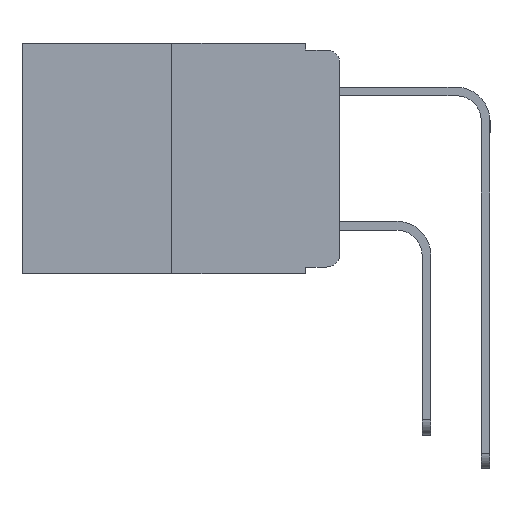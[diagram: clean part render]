
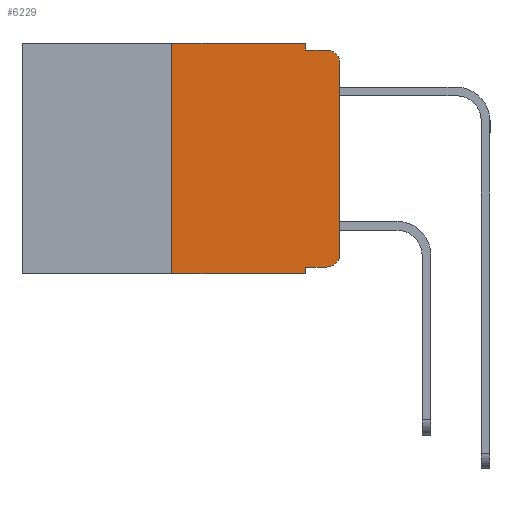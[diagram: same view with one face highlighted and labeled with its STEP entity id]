
A CAD part, left-side view. The second image highlights one B-rep face of the part: STEP entity #6229.
In plain terms, the highlighted planar face has unit normal (-1, 0, 0).
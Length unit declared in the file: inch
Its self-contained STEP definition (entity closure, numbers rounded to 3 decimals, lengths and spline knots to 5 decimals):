
#60 = LINE ( 'NONE', #8487, #2814 ) ;
#411 = CARTESIAN_POINT ( 'NONE',  ( 0., 0.051, 0. ) ) ;
#738 = VECTOR ( 'NONE', #11213, 39.37008 ) ;
#787 = LINE ( 'NONE', #5818, #11180 ) ;
#874 = VERTEX_POINT ( 'NONE', #4014 ) ;
#1702 = ORIENTED_EDGE ( 'NONE', *, *, #7614, .F. ) ;
#1837 = DIRECTION ( 'NONE',  ( 0., -1., 0. ) ) ;
#1943 = ORIENTED_EDGE ( 'NONE', *, *, #8158, .F. ) ;
#2153 = DIRECTION ( 'NONE',  ( -1., 0., 0. ) ) ;
#2157 = CARTESIAN_POINT ( 'NONE',  ( 0., 0.02, -0.313 ) ) ;
#2198 = VERTEX_POINT ( 'NONE', #11576 ) ;
#2254 = AXIS2_PLACEMENT_3D ( 'NONE', #2157, #2153, #7334 ) ;
#2568 = ORIENTED_EDGE ( 'NONE', *, *, #8787, .F. ) ;
#2718 = ORIENTED_EDGE ( 'NONE', *, *, #9381, .T. ) ;
#2744 = FACE_OUTER_BOUND ( 'NONE', #4644, .T. ) ;
#2746 = ORIENTED_EDGE ( 'NONE', *, *, #10650, .T. ) ;
#2813 = VERTEX_POINT ( 'NONE', #5570 ) ;
#2814 = VECTOR ( 'NONE', #6562, 39.37008 ) ;
#3187 = VECTOR ( 'NONE', #11458, 39.37008 ) ;
#3486 = LINE ( 'NONE', #411, #3187 ) ;
#3509 = VERTEX_POINT ( 'NONE', #10684 ) ;
#3555 = CARTESIAN_POINT ( 'NONE',  ( 0., 0., 0. ) ) ;
#4014 = CARTESIAN_POINT ( 'NONE',  ( 0., 0.051, -0.333 ) ) ;
#4319 = CARTESIAN_POINT ( 'NONE',  ( 0., 0.25, 0. ) ) ;
#4393 = LINE ( 'NONE', #7600, #7056 ) ;
#4644 = EDGE_LOOP ( 'NONE', ( #2746, #2718, #2568, #1943, #1702, #10249, #6301, #6233, #5969, #11998 ) ) ;
#4831 = CARTESIAN_POINT ( 'NONE',  ( 0., 0.051, -0.343 ) ) ;
#5222 = VERTEX_POINT ( 'NONE', #11667 ) ;
#5246 = PLANE ( 'NONE',  #8975 ) ;
#5377 = VECTOR ( 'NONE', #11049, 39.37008 ) ;
#5530 = CARTESIAN_POINT ( 'NONE',  ( 0., 0.051, 0. ) ) ;
#5541 = CARTESIAN_POINT ( 'NONE',  ( 0., 0.02, -0.03 ) ) ;
#5548 = EDGE_CURVE ( 'NONE', #5684, #2813, #10314, .T. ) ;
#5570 = CARTESIAN_POINT ( 'NONE',  ( 0., 0., -0.313 ) ) ;
#5634 = DIRECTION ( 'NONE',  ( 0., -1., 0. ) ) ;
#5684 = VERTEX_POINT ( 'NONE', #7841 ) ;
#5818 = CARTESIAN_POINT ( 'NONE',  ( 0., 0.473, -0.343 ) ) ;
#5872 = DIRECTION ( 'NONE',  ( 1., 0., 0. ) ) ;
#5935 = VERTEX_POINT ( 'NONE', #9921 ) ;
#5969 = ORIENTED_EDGE ( 'NONE', *, *, #6231, .T. ) ;
#5975 = VECTOR ( 'NONE', #10087, 39.37008 ) ;
#6063 = DIRECTION ( 'NONE',  ( 0., 0., -1. ) ) ;
#6110 = LINE ( 'NONE', #5530, #738 ) ;
#6229 = ADVANCED_FACE ( 'NONE', ( #2744 ), #5246, .F. ) ;
#6231 = EDGE_CURVE ( 'NONE', #874, #5684, #7674, .T. ) ;
#6233 = ORIENTED_EDGE ( 'NONE', *, *, #6895, .F. ) ;
#6301 = ORIENTED_EDGE ( 'NONE', *, *, #11462, .T. ) ;
#6389 = AXIS2_PLACEMENT_3D ( 'NONE', #5541, #12167, #6550 ) ;
#6550 = DIRECTION ( 'NONE',  ( 0., 0., -1. ) ) ;
#6562 = DIRECTION ( 'NONE',  ( 0., -1., 0. ) ) ;
#6895 = EDGE_CURVE ( 'NONE', #874, #10151, #3486, .T. ) ;
#7022 = CARTESIAN_POINT ( 'NONE',  ( 0., 0.473, 0. ) ) ;
#7056 = VECTOR ( 'NONE', #5634, 39.37008 ) ;
#7334 = DIRECTION ( 'NONE',  ( 0., 0., -1. ) ) ;
#7525 = EDGE_CURVE ( 'NONE', #5222, #2198, #8231, .T. ) ;
#7600 = CARTESIAN_POINT ( 'NONE',  ( 0., 0.473, 0. ) ) ;
#7614 = EDGE_CURVE ( 'NONE', #2198, #9263, #4393, .T. ) ;
#7674 = LINE ( 'NONE', #10994, #5377 ) ;
#7840 = VECTOR ( 'NONE', #12188, 39.37008 ) ;
#7841 = CARTESIAN_POINT ( 'NONE',  ( 0., 0.02, -0.333 ) ) ;
#8158 = EDGE_CURVE ( 'NONE', #9263, #3509, #6110, .T. ) ;
#8231 = LINE ( 'NONE', #4319, #5975 ) ;
#8487 = CARTESIAN_POINT ( 'NONE',  ( 0., 0.051, -0.01 ) ) ;
#8787 = EDGE_CURVE ( 'NONE', #3509, #5935, #60, .T. ) ;
#8975 = AXIS2_PLACEMENT_3D ( 'NONE', #7022, #5872, #6063 ) ;
#9263 = VERTEX_POINT ( 'NONE', #10125 ) ;
#9381 = EDGE_CURVE ( 'NONE', #9662, #5935, #10050, .T. ) ;
#9662 = VERTEX_POINT ( 'NONE', #10696 ) ;
#9921 = CARTESIAN_POINT ( 'NONE',  ( 0., 0.02, -0.01 ) ) ;
#10050 = CIRCLE ( 'NONE', #6389, 0.02 ) ;
#10087 = DIRECTION ( 'NONE',  ( 0., 0., 1. ) ) ;
#10125 = CARTESIAN_POINT ( 'NONE',  ( 0., 0.051, 0. ) ) ;
#10151 = VERTEX_POINT ( 'NONE', #4831 ) ;
#10249 = ORIENTED_EDGE ( 'NONE', *, *, #7525, .F. ) ;
#10313 = LINE ( 'NONE', #3555, #7840 ) ;
#10314 = CIRCLE ( 'NONE', #2254, 0.02 ) ;
#10650 = EDGE_CURVE ( 'NONE', #2813, #9662, #10313, .T. ) ;
#10684 = CARTESIAN_POINT ( 'NONE',  ( 0., 0.051, -0.01 ) ) ;
#10696 = CARTESIAN_POINT ( 'NONE',  ( 0., 0., -0.03 ) ) ;
#10994 = CARTESIAN_POINT ( 'NONE',  ( 0., 0.051, -0.333 ) ) ;
#11049 = DIRECTION ( 'NONE',  ( 0., -1., 0. ) ) ;
#11180 = VECTOR ( 'NONE', #1837, 39.37008 ) ;
#11213 = DIRECTION ( 'NONE',  ( 0., 0., -1. ) ) ;
#11458 = DIRECTION ( 'NONE',  ( 0., 0., -1. ) ) ;
#11462 = EDGE_CURVE ( 'NONE', #5222, #10151, #787, .T. ) ;
#11576 = CARTESIAN_POINT ( 'NONE',  ( 0., 0.25, 0. ) ) ;
#11667 = CARTESIAN_POINT ( 'NONE',  ( 0., 0.25, -0.343 ) ) ;
#11998 = ORIENTED_EDGE ( 'NONE', *, *, #5548, .T. ) ;
#12167 = DIRECTION ( 'NONE',  ( -1., 0., 0. ) ) ;
#12188 = DIRECTION ( 'NONE',  ( 0., 0., 1. ) ) ;
